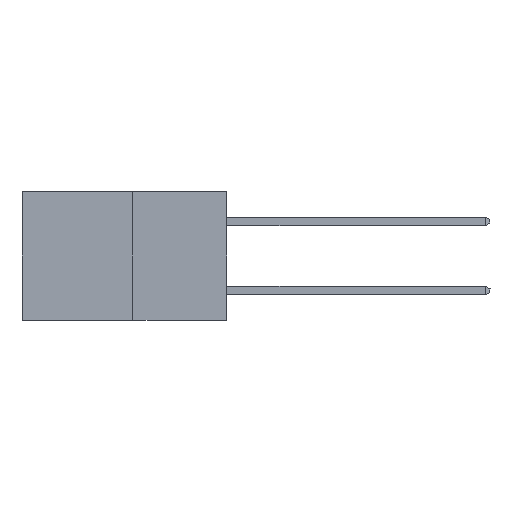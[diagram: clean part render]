
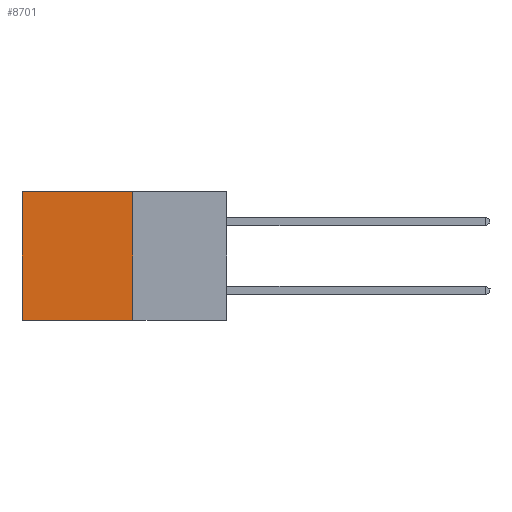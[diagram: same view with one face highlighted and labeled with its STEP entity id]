
A CAD part, left-side view. The second image highlights one B-rep face of the part: STEP entity #8701.
In plain terms, the highlighted planar face has unit normal (-1, 0, 0).
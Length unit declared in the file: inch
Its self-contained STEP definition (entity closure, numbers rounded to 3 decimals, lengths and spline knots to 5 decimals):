
#138 = EDGE_CURVE ( 'NONE', #7418, #4244, #4273, .T. ) ;
#206 = VECTOR ( 'NONE', #6447, 39.37008 ) ;
#734 = ORIENTED_EDGE ( 'NONE', *, *, #3947, .T. ) ;
#1042 = DIRECTION ( 'NONE',  ( 0., 0., -1. ) ) ;
#1624 = CARTESIAN_POINT ( 'NONE',  ( 0.277, 0.27, -0.37 ) ) ;
#1863 = ORIENTED_EDGE ( 'NONE', *, *, #8653, .F. ) ;
#2788 = CARTESIAN_POINT ( 'NONE',  ( 0.277, 0.59, -0.37 ) ) ;
#2894 = CARTESIAN_POINT ( 'NONE',  ( 0.277, 0.27, 0. ) ) ;
#2895 = DIRECTION ( 'NONE',  ( 0., 0., -1. ) ) ;
#3244 = ORIENTED_EDGE ( 'NONE', *, *, #5763, .F. ) ;
#3525 = CARTESIAN_POINT ( 'NONE',  ( 0.277, 0.59, -0.37 ) ) ;
#3947 = EDGE_CURVE ( 'NONE', #6842, #7418, #7163, .T. ) ;
#3956 = LINE ( 'NONE', #1624, #7336 ) ;
#4155 = DIRECTION ( 'NONE',  ( 0., 1., 0. ) ) ;
#4202 = CARTESIAN_POINT ( 'NONE',  ( 0.277, 0.27, -0.37 ) ) ;
#4244 = VERTEX_POINT ( 'NONE', #2788 ) ;
#4273 = LINE ( 'NONE', #3525, #7444 ) ;
#4422 = VECTOR ( 'NONE', #4155, 39.37008 ) ;
#4932 = CARTESIAN_POINT ( 'NONE',  ( 0.277, 0.27, -0.37 ) ) ;
#5053 = CARTESIAN_POINT ( 'NONE',  ( 0.277, 0.27, 0. ) ) ;
#5502 = AXIS2_PLACEMENT_3D ( 'NONE', #4202, #6923, #2895 ) ;
#5506 = CARTESIAN_POINT ( 'NONE',  ( 0.277, 0.27, -0.37 ) ) ;
#5763 = EDGE_CURVE ( 'NONE', #6842, #6866, #3956, .T. ) ;
#6000 = FACE_OUTER_BOUND ( 'NONE', #7928, .T. ) ;
#6251 = PLANE ( 'NONE',  #5502 ) ;
#6432 = LINE ( 'NONE', #5506, #4422 ) ;
#6447 = DIRECTION ( 'NONE',  ( 0., 1., 0. ) ) ;
#6842 = VERTEX_POINT ( 'NONE', #2894 ) ;
#6866 = VERTEX_POINT ( 'NONE', #4932 ) ;
#6923 = DIRECTION ( 'NONE',  ( 1., 0., 0. ) ) ;
#7163 = LINE ( 'NONE', #5053, #206 ) ;
#7336 = VECTOR ( 'NONE', #1042, 39.37008 ) ;
#7418 = VERTEX_POINT ( 'NONE', #7507 ) ;
#7444 = VECTOR ( 'NONE', #8354, 39.37008 ) ;
#7507 = CARTESIAN_POINT ( 'NONE',  ( 0.277, 0.59, 0. ) ) ;
#7805 = ORIENTED_EDGE ( 'NONE', *, *, #138, .T. ) ;
#7928 = EDGE_LOOP ( 'NONE', ( #7805, #1863, #3244, #734 ) ) ;
#8354 = DIRECTION ( 'NONE',  ( 0., 0., -1. ) ) ;
#8653 = EDGE_CURVE ( 'NONE', #6866, #4244, #6432, .T. ) ;
#8701 = ADVANCED_FACE ( 'NONE', ( #6000 ), #6251, .F. ) ;
